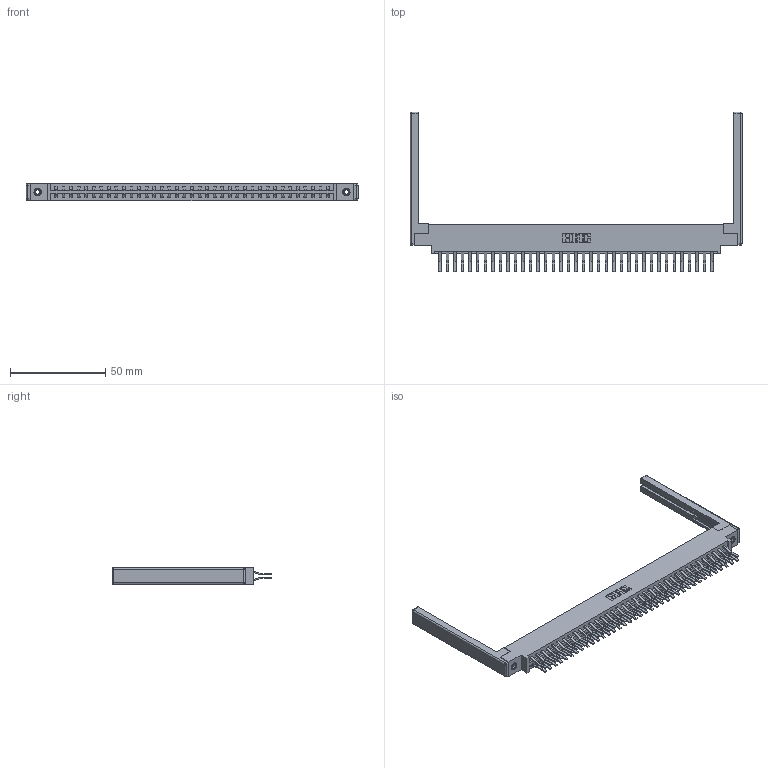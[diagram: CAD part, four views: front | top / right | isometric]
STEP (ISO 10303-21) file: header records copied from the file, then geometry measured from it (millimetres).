
FILE_DESCRIPTION (( 'STEP AP203' ), '1' );
FILE_NAME ('337-074-560-868.STEP', '2019-10-15T12:58:08', ( '' ), ( '' ), 'SwSTEP 2.0', 'SolidWorks 2016', '' );
FILE_SCHEMA (( 'CONFIG_CONTROL_DESIGN' ));
Length unit declared in the file: inch
Products named in the file (5): 307-220-068; 345-292-001_560 Tail; 337 Part_0.170 Offset - 0.156 Dia-TI; 337-074-560-868; 345-250-001_345-250-001-102
Assembly tree (79 placements, depth 2):
  337-074-560-868
    337 Part_0.170 Offset - 0.156 Dia-TI
    345-292-001_560 Tail  x74
    345-250-001_345-250-001-102  x2
    307-220-068  x2
Bounding box: 174.04 x 83.84 x 9.4 mm (x, y, z)
Volume: 23027.6 mm3; surface area: 26573.2 mm2
Topology: 79 solids, 79 shells, 4416 faces, 13071 edges, 8594 vertices
Faces by surface type: plane 2974, cylinder 1418, cone 12, sphere 8, torus 4
Entity records: 32314 total; most frequent: CARTESIAN_POINT 5415, ORIENTED_EDGE 5340, DIRECTION 4688, EDGE_CURVE 2670, VECTOR 2488, LINE 2488, VERTEX_POINT 1770, AXIS2_PLACEMENT_3D 1100
